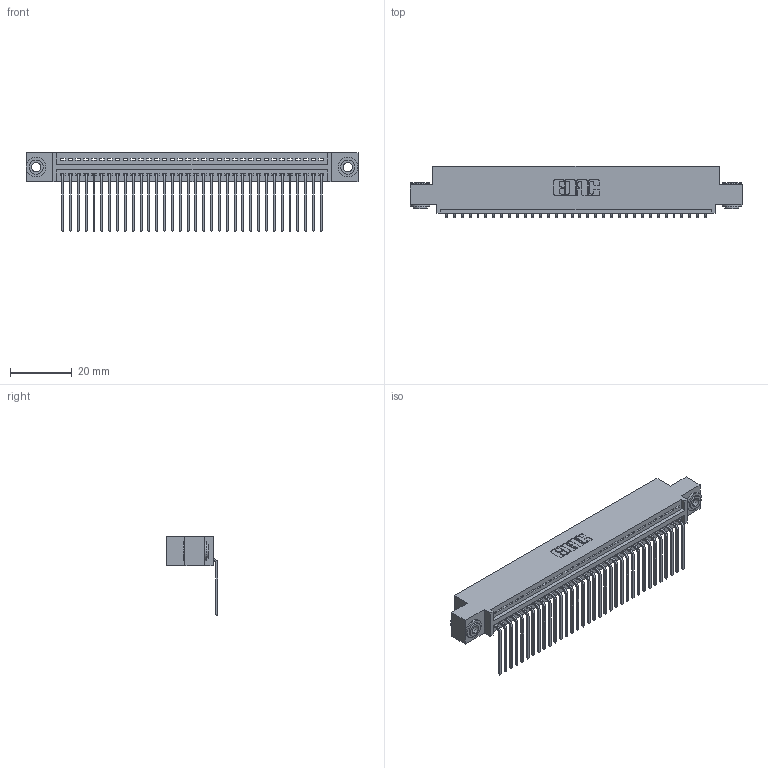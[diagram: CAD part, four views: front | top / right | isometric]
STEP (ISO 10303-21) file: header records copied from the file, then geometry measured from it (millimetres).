
FILE_DESCRIPTION (( 'STEP AP203' ), '1' );
FILE_NAME ('395-034-559-403.STEP', '2018-11-13T10:43:38', ( '' ), ( '' ), 'SwSTEP 2.0', 'SolidWorks 2016', '' );
FILE_SCHEMA (( 'CONFIG_CONTROL_DESIGN' ));
Length unit declared in the file: inch
Products named in the file (4): 395-034-559-403; 345 Part_0.110 Offset - 0.156 Dia-TH; 345-292-001_558 559 Tail - 1; 345-250-002_345-250-002-102
Assembly tree (37 placements, depth 2):
  395-034-559-403
    345 Part_0.110 Offset - 0.156 Dia-TH
    345-292-001_558 559 Tail - 1  x34
    345-250-002_345-250-002-102  x2
Bounding box: 107.57 x 16.75 x 25.53 mm (x, y, z)
Volume: 10210.8 mm3; surface area: 14422.5 mm2
Topology: 37 solids, 37 shells, 2208 faces, 6617 edges, 4362 vertices
Faces by surface type: plane 1522, cylinder 678, cone 8
Entity records: 27532 total; most frequent: CARTESIAN_POINT 4749, ORIENTED_EDGE 4710, DIRECTION 4189, EDGE_CURVE 2355, VECTOR 2063, LINE 2063, VERTEX_POINT 1566, AXIS2_PLACEMENT_3D 1063
